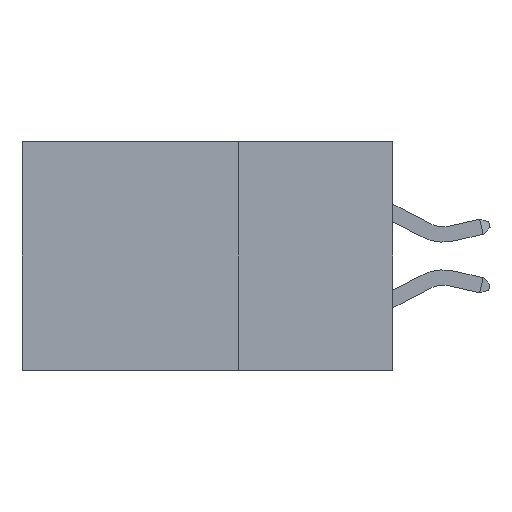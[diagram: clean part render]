
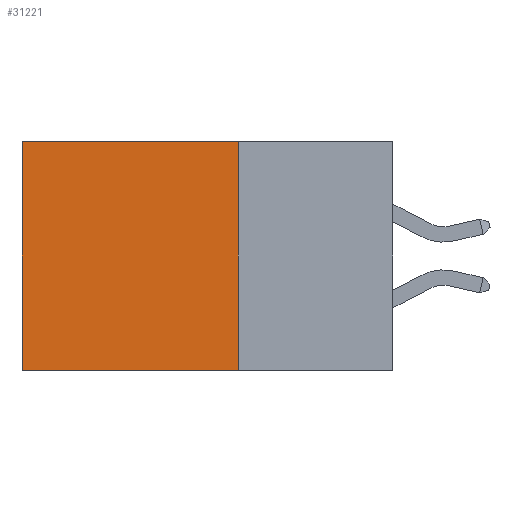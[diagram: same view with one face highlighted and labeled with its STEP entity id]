
A CAD part, left-side view. The second image highlights one B-rep face of the part: STEP entity #31221.
In plain terms, the highlighted planar face has unit normal (-1, 0, 0).
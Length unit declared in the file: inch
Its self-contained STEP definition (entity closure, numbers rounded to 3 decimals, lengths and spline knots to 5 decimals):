
#403 = DIRECTION ( 'NONE',  ( 0., 1., 0. ) ) ;
#578 = LINE ( 'NONE', #16420, #25244 ) ;
#1985 = DIRECTION ( 'NONE',  ( 0., 1., 0. ) ) ;
#2607 = EDGE_CURVE ( 'NONE', #6832, #31348, #19730, .T. ) ;
#3317 = CARTESIAN_POINT ( 'NONE',  ( 0.2875, 0.25, -0.37 ) ) ;
#3656 = AXIS2_PLACEMENT_3D ( 'NONE', #9427, #9929, #32917 ) ;
#6832 = VERTEX_POINT ( 'NONE', #12445 ) ;
#7382 = LINE ( 'NONE', #17917, #15280 ) ;
#8699 = ORIENTED_EDGE ( 'NONE', *, *, #11114, .T. ) ;
#9427 = CARTESIAN_POINT ( 'NONE',  ( 0.2875, 0.25, 0. ) ) ;
#9929 = DIRECTION ( 'NONE',  ( 1., 0., 0. ) ) ;
#10091 = PLANE ( 'NONE',  #3656 ) ;
#10887 = EDGE_LOOP ( 'NONE', ( #31911, #33008, #14439, #8699 ) ) ;
#11114 = EDGE_CURVE ( 'NONE', #32573, #6832, #578, .T. ) ;
#12445 = CARTESIAN_POINT ( 'NONE',  ( 0.2875, 0.6, 0. ) ) ;
#12683 = LINE ( 'NONE', #15073, #19461 ) ;
#14439 = ORIENTED_EDGE ( 'NONE', *, *, #17126, .F. ) ;
#15073 = CARTESIAN_POINT ( 'NONE',  ( 0.2875, 0.25, -0.37 ) ) ;
#15280 = VECTOR ( 'NONE', #23364, 39.37008 ) ;
#16420 = CARTESIAN_POINT ( 'NONE',  ( 0.2875, 0.25, 0. ) ) ;
#17126 = EDGE_CURVE ( 'NONE', #32573, #32821, #7382, .T. ) ;
#17917 = CARTESIAN_POINT ( 'NONE',  ( 0.2875, 0.25, 0. ) ) ;
#19461 = VECTOR ( 'NONE', #1985, 39.37008 ) ;
#19730 = LINE ( 'NONE', #27582, #32491 ) ;
#23364 = DIRECTION ( 'NONE',  ( 0., 0., -1. ) ) ;
#25244 = VECTOR ( 'NONE', #403, 39.37008 ) ;
#26371 = EDGE_CURVE ( 'NONE', #32821, #31348, #12683, .T. ) ;
#27582 = CARTESIAN_POINT ( 'NONE',  ( 0.2875, 0.6, 0. ) ) ;
#28167 = FACE_OUTER_BOUND ( 'NONE', #10887, .T. ) ;
#30532 = CARTESIAN_POINT ( 'NONE',  ( 0.2875, 0.6, -0.37 ) ) ;
#30622 = DIRECTION ( 'NONE',  ( 0., 0., -1. ) ) ;
#31221 = ADVANCED_FACE ( 'NONE', ( #28167 ), #10091, .F. ) ;
#31348 = VERTEX_POINT ( 'NONE', #30532 ) ;
#31911 = ORIENTED_EDGE ( 'NONE', *, *, #2607, .T. ) ;
#32135 = CARTESIAN_POINT ( 'NONE',  ( 0.2875, 0.25, 0. ) ) ;
#32491 = VECTOR ( 'NONE', #30622, 39.37008 ) ;
#32573 = VERTEX_POINT ( 'NONE', #32135 ) ;
#32821 = VERTEX_POINT ( 'NONE', #3317 ) ;
#32917 = DIRECTION ( 'NONE',  ( 0., 0., -1. ) ) ;
#33008 = ORIENTED_EDGE ( 'NONE', *, *, #26371, .F. ) ;
